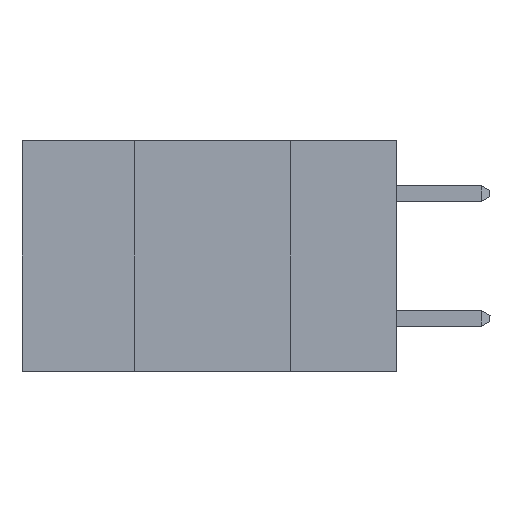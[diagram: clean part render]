
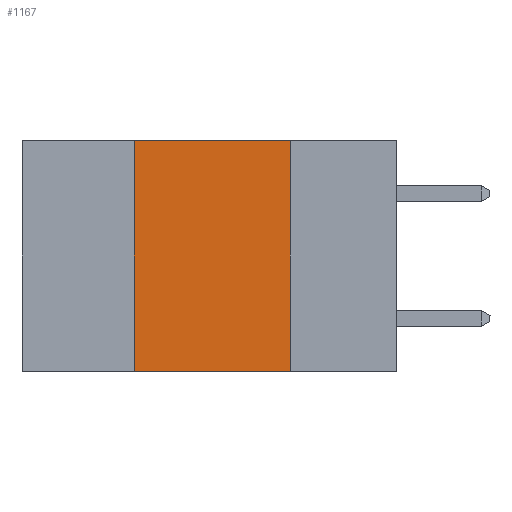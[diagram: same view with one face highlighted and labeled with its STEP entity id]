
A CAD part, left-side view. The second image highlights one B-rep face of the part: STEP entity #1167.
In plain terms, the highlighted planar face has unit normal (-1, 0, 0).
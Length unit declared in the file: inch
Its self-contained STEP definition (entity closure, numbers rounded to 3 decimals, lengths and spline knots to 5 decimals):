
#18 = FACE_OUTER_BOUND ( 'NONE', #681, .T. ) ;
#246 = EDGE_CURVE ( 'NONE', #2151, #9671, #3362, .T. ) ;
#277 = ORIENTED_EDGE ( 'NONE', *, *, #14336, .F. ) ;
#298 = CARTESIAN_POINT ( 'NONE',  ( 0., 0.42, -0.37 ) ) ;
#681 = EDGE_LOOP ( 'NONE', ( #11781, #15106, #277, #4564 ) ) ;
#957 = CARTESIAN_POINT ( 'NONE',  ( 0., 0.17, 0. ) ) ;
#1167 = ADVANCED_FACE ( 'NONE', ( #18 ), #11573, .F. ) ;
#1415 = VECTOR ( 'NONE', #14942, 39.37008 ) ;
#2151 = VERTEX_POINT ( 'NONE', #10877 ) ;
#2155 = VERTEX_POINT ( 'NONE', #298 ) ;
#2785 = CARTESIAN_POINT ( 'NONE',  ( 0., 0.17, -0.37 ) ) ;
#2914 = DIRECTION ( 'NONE',  ( 0., -1., 0. ) ) ;
#3179 = VECTOR ( 'NONE', #10932, 39.37008 ) ;
#3362 = LINE ( 'NONE', #9795, #3179 ) ;
#4157 = CARTESIAN_POINT ( 'NONE',  ( 0., 0.17, 0. ) ) ;
#4529 = LINE ( 'NONE', #4157, #1415 ) ;
#4564 = ORIENTED_EDGE ( 'NONE', *, *, #10069, .T. ) ;
#4690 = DIRECTION ( 'NONE',  ( 0., 0., -1. ) ) ;
#5072 = VERTEX_POINT ( 'NONE', #2785 ) ;
#6477 = CARTESIAN_POINT ( 'NONE',  ( 0., 0.6, -0.37 ) ) ;
#6765 = VECTOR ( 'NONE', #7767, 39.37008 ) ;
#6856 = CARTESIAN_POINT ( 'NONE',  ( 0., 0.6, 0. ) ) ;
#7757 = LINE ( 'NONE', #6477, #10905 ) ;
#7767 = DIRECTION ( 'NONE',  ( 0., 0., 1. ) ) ;
#9671 = VERTEX_POINT ( 'NONE', #957 ) ;
#9795 = CARTESIAN_POINT ( 'NONE',  ( 0., 0.6, 0. ) ) ;
#9927 = LINE ( 'NONE', #14839, #6765 ) ;
#10069 = EDGE_CURVE ( 'NONE', #2155, #5072, #7757, .T. ) ;
#10877 = CARTESIAN_POINT ( 'NONE',  ( 0., 0.42, 0. ) ) ;
#10905 = VECTOR ( 'NONE', #2914, 39.37008 ) ;
#10932 = DIRECTION ( 'NONE',  ( 0., -1., 0. ) ) ;
#11573 = PLANE ( 'NONE',  #15121 ) ;
#11781 = ORIENTED_EDGE ( 'NONE', *, *, #15179, .F. ) ;
#14336 = EDGE_CURVE ( 'NONE', #2155, #2151, #9927, .T. ) ;
#14839 = CARTESIAN_POINT ( 'NONE',  ( 0., 0.42, 0. ) ) ;
#14942 = DIRECTION ( 'NONE',  ( 0., 0., -1. ) ) ;
#15106 = ORIENTED_EDGE ( 'NONE', *, *, #246, .F. ) ;
#15121 = AXIS2_PLACEMENT_3D ( 'NONE', #6856, #15137, #4690 ) ;
#15137 = DIRECTION ( 'NONE',  ( 1., 0., 0. ) ) ;
#15179 = EDGE_CURVE ( 'NONE', #9671, #5072, #4529, .T. ) ;
